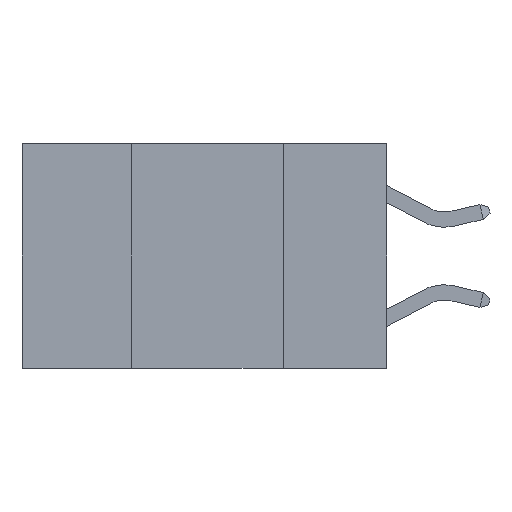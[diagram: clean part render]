
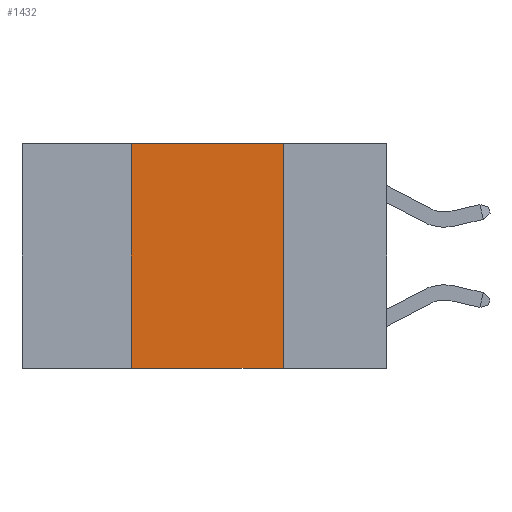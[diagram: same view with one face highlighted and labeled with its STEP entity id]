
A CAD part, left-side view. The second image highlights one B-rep face of the part: STEP entity #1432.
In plain terms, the highlighted planar face has unit normal (-1, 0, 0).
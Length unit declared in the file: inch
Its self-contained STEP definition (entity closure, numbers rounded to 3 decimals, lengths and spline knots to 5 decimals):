
#680 = LINE ( 'NONE', #983, #5374 ) ;
#983 = CARTESIAN_POINT ( 'NONE',  ( 0., 0.17, 0. ) ) ;
#1206 = PLANE ( 'NONE',  #5697 ) ;
#1432 = ADVANCED_FACE ( 'NONE', ( #7197 ), #1206, .F. ) ;
#1725 = DIRECTION ( 'NONE',  ( 0., 0., 1. ) ) ;
#1890 = VECTOR ( 'NONE', #6901, 39.37008 ) ;
#2589 = CARTESIAN_POINT ( 'NONE',  ( 0., 0.6, 0. ) ) ;
#2707 = CARTESIAN_POINT ( 'NONE',  ( 0., 0.42, 0. ) ) ;
#2804 = CARTESIAN_POINT ( 'NONE',  ( 0., 0.42, 0. ) ) ;
#2941 = EDGE_CURVE ( 'NONE', #6421, #7149, #3477, .T. ) ;
#3477 = LINE ( 'NONE', #10512, #1890 ) ;
#3695 = LINE ( 'NONE', #2707, #6506 ) ;
#4418 = EDGE_LOOP ( 'NONE', ( #11114, #9290, #9019, #10137 ) ) ;
#4841 = DIRECTION ( 'NONE',  ( 0., -1., 0. ) ) ;
#5027 = VERTEX_POINT ( 'NONE', #2804 ) ;
#5374 = VECTOR ( 'NONE', #7528, 39.37008 ) ;
#5697 = AXIS2_PLACEMENT_3D ( 'NONE', #2589, #7610, #10444 ) ;
#5826 = CARTESIAN_POINT ( 'NONE',  ( 0., 0.42, -0.37 ) ) ;
#5963 = VERTEX_POINT ( 'NONE', #10746 ) ;
#6277 = VECTOR ( 'NONE', #4841, 39.37008 ) ;
#6421 = VERTEX_POINT ( 'NONE', #5826 ) ;
#6506 = VECTOR ( 'NONE', #1725, 39.37008 ) ;
#6901 = DIRECTION ( 'NONE',  ( 0., -1., 0. ) ) ;
#7149 = VERTEX_POINT ( 'NONE', #9215 ) ;
#7197 = FACE_OUTER_BOUND ( 'NONE', #4418, .T. ) ;
#7528 = DIRECTION ( 'NONE',  ( 0., 0., -1. ) ) ;
#7610 = DIRECTION ( 'NONE',  ( 1., 0., 0. ) ) ;
#7757 = EDGE_CURVE ( 'NONE', #6421, #5027, #3695, .T. ) ;
#8537 = CARTESIAN_POINT ( 'NONE',  ( 0., 0.6, 0. ) ) ;
#9019 = ORIENTED_EDGE ( 'NONE', *, *, #7757, .F. ) ;
#9034 = LINE ( 'NONE', #8537, #6277 ) ;
#9215 = CARTESIAN_POINT ( 'NONE',  ( 0., 0.17, -0.37 ) ) ;
#9290 = ORIENTED_EDGE ( 'NONE', *, *, #10283, .F. ) ;
#10137 = ORIENTED_EDGE ( 'NONE', *, *, #2941, .T. ) ;
#10283 = EDGE_CURVE ( 'NONE', #5027, #5963, #9034, .T. ) ;
#10444 = DIRECTION ( 'NONE',  ( 0., 0., -1. ) ) ;
#10512 = CARTESIAN_POINT ( 'NONE',  ( 0., 0.6, -0.37 ) ) ;
#10717 = EDGE_CURVE ( 'NONE', #5963, #7149, #680, .T. ) ;
#10746 = CARTESIAN_POINT ( 'NONE',  ( 0., 0.17, 0. ) ) ;
#11114 = ORIENTED_EDGE ( 'NONE', *, *, #10717, .F. ) ;
